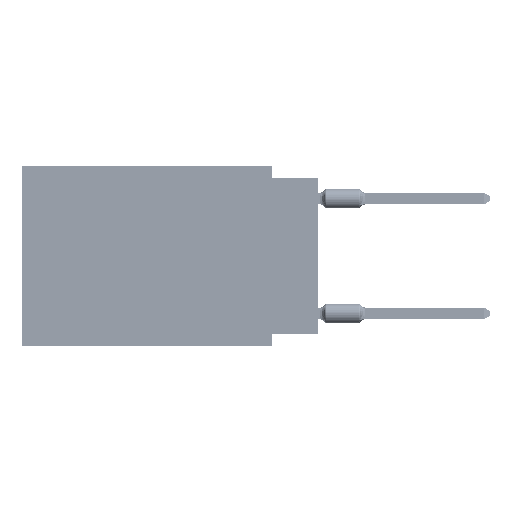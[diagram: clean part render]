
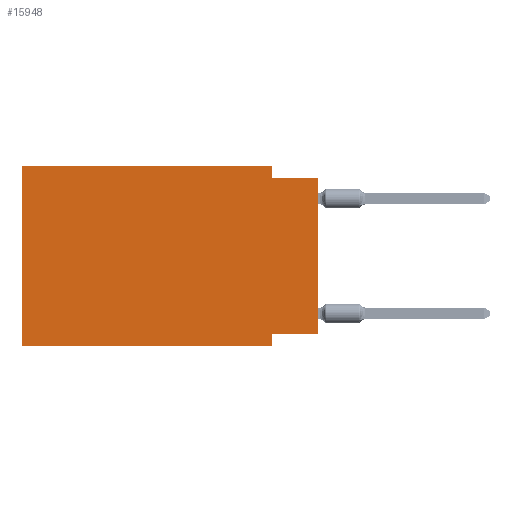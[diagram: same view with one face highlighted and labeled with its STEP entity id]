
A CAD part, left-side view. The second image highlights one B-rep face of the part: STEP entity #15948.
In plain terms, the highlighted planar face has unit normal (-1, 0, 0).
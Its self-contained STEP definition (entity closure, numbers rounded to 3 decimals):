
#160 = CARTESIAN_POINT ( 'NONE',  ( 0., 0., -0.635 ) ) ;
#4522 = CARTESIAN_POINT ( 'NONE',  ( 0., 16.383, 0. ) ) ;
#5381 = CARTESIAN_POINT ( 'NONE',  ( 0., 16.383, 0. ) ) ;
#5715 = DIRECTION ( 'NONE',  ( 0., -1., 0. ) ) ;
#6021 = VECTOR ( 'NONE', #55479, 1000. ) ;
#6768 = ORIENTED_EDGE ( 'NONE', *, *, #44002, .F. ) ;
#6849 = ORIENTED_EDGE ( 'NONE', *, *, #9124, .F. ) ;
#8456 = LINE ( 'NONE', #20198, #6021 ) ;
#8547 = CARTESIAN_POINT ( 'NONE',  ( 0., 2.54, -0.635 ) ) ;
#8705 = AXIS2_PLACEMENT_3D ( 'NONE', #5381, #53200, #39228 ) ;
#9124 = EDGE_CURVE ( 'NONE', #54401, #75551, #42579, .T. ) ;
#15082 = CARTESIAN_POINT ( 'NONE',  ( 0., 0., -9.271 ) ) ;
#15948 = ADVANCED_FACE ( 'NONE', ( #58695 ), #38837, .F. ) ;
#18125 = LINE ( 'NONE', #40870, #38479 ) ;
#18279 = CARTESIAN_POINT ( 'NONE',  ( 0., 2.54, 0. ) ) ;
#19780 = ORIENTED_EDGE ( 'NONE', *, *, #25384, .F. ) ;
#20198 = CARTESIAN_POINT ( 'NONE',  ( 0., 2.54, -9.906 ) ) ;
#22060 = VECTOR ( 'NONE', #72328, 1000. ) ;
#25228 = EDGE_CURVE ( 'NONE', #67931, #31620, #34319, .T. ) ;
#25384 = EDGE_CURVE ( 'NONE', #35649, #77270, #52724, .T. ) ;
#26536 = CARTESIAN_POINT ( 'NONE',  ( 0., 0., -0.635 ) ) ;
#27300 = VERTEX_POINT ( 'NONE', #68183 ) ;
#27854 = CARTESIAN_POINT ( 'NONE',  ( 0., 16.383, -9.906 ) ) ;
#29594 = CARTESIAN_POINT ( 'NONE',  ( 0., 0., -9.271 ) ) ;
#30759 = CARTESIAN_POINT ( 'NONE',  ( 0., 16.383, 0. ) ) ;
#31620 = VERTEX_POINT ( 'NONE', #57755 ) ;
#32325 = EDGE_CURVE ( 'NONE', #75551, #38111, #32416, .T. ) ;
#32416 = LINE ( 'NONE', #26536, #66890 ) ;
#34319 = LINE ( 'NONE', #4522, #49952 ) ;
#35649 = VERTEX_POINT ( 'NONE', #15082 ) ;
#36242 = ORIENTED_EDGE ( 'NONE', *, *, #41493, .T. ) ;
#38111 = VERTEX_POINT ( 'NONE', #160 ) ;
#38479 = VECTOR ( 'NONE', #60071, 1000. ) ;
#38837 = PLANE ( 'NONE',  #8705 ) ;
#39228 = DIRECTION ( 'NONE',  ( 0., 0., -1. ) ) ;
#39966 = EDGE_CURVE ( 'NONE', #67931, #27300, #53314, .T. ) ;
#40870 = CARTESIAN_POINT ( 'NONE',  ( 0., 0., 0. ) ) ;
#41493 = EDGE_CURVE ( 'NONE', #35649, #38111, #18125, .T. ) ;
#42509 = VECTOR ( 'NONE', #70703, 1000. ) ;
#42579 = LINE ( 'NONE', #18279, #22060 ) ;
#42901 = DIRECTION ( 'NONE',  ( 0., -1., 0. ) ) ;
#42920 = CARTESIAN_POINT ( 'NONE',  ( 0., 2.54, 0. ) ) ;
#43473 = EDGE_CURVE ( 'NONE', #31620, #54401, #65632, .T. ) ;
#44002 = EDGE_CURVE ( 'NONE', #77270, #27300, #8456, .T. ) ;
#44221 = EDGE_LOOP ( 'NONE', ( #36242, #47042, #6849, #64050, #60270, #73308, #6768, #19780 ) ) ;
#46259 = DIRECTION ( 'NONE',  ( 0., -1., 0. ) ) ;
#47042 = ORIENTED_EDGE ( 'NONE', *, *, #32325, .F. ) ;
#49563 = VECTOR ( 'NONE', #46259, 1000. ) ;
#49952 = VECTOR ( 'NONE', #69568, 1000. ) ;
#51172 = CARTESIAN_POINT ( 'NONE',  ( 0., 2.54, -9.271 ) ) ;
#52724 = LINE ( 'NONE', #29594, #42509 ) ;
#53200 = DIRECTION ( 'NONE',  ( 1., 0., 0. ) ) ;
#53314 = LINE ( 'NONE', #27854, #49563 ) ;
#54401 = VERTEX_POINT ( 'NONE', #42920 ) ;
#55479 = DIRECTION ( 'NONE',  ( 0., 0., -1. ) ) ;
#57755 = CARTESIAN_POINT ( 'NONE',  ( 0., 16.383, 0. ) ) ;
#58695 = FACE_OUTER_BOUND ( 'NONE', #44221, .T. ) ;
#60071 = DIRECTION ( 'NONE',  ( 0., 0., 1. ) ) ;
#60270 = ORIENTED_EDGE ( 'NONE', *, *, #25228, .F. ) ;
#64050 = ORIENTED_EDGE ( 'NONE', *, *, #43473, .F. ) ;
#65632 = LINE ( 'NONE', #30759, #67266 ) ;
#66890 = VECTOR ( 'NONE', #5715, 1000. ) ;
#67266 = VECTOR ( 'NONE', #42901, 1000. ) ;
#67931 = VERTEX_POINT ( 'NONE', #75222 ) ;
#68183 = CARTESIAN_POINT ( 'NONE',  ( 0., 2.54, -9.906 ) ) ;
#69568 = DIRECTION ( 'NONE',  ( 0., 0., 1. ) ) ;
#70703 = DIRECTION ( 'NONE',  ( 0., 1., 0. ) ) ;
#72328 = DIRECTION ( 'NONE',  ( 0., 0., -1. ) ) ;
#73308 = ORIENTED_EDGE ( 'NONE', *, *, #39966, .T. ) ;
#75222 = CARTESIAN_POINT ( 'NONE',  ( 0., 16.383, -9.906 ) ) ;
#75551 = VERTEX_POINT ( 'NONE', #8547 ) ;
#77270 = VERTEX_POINT ( 'NONE', #51172 ) ;
